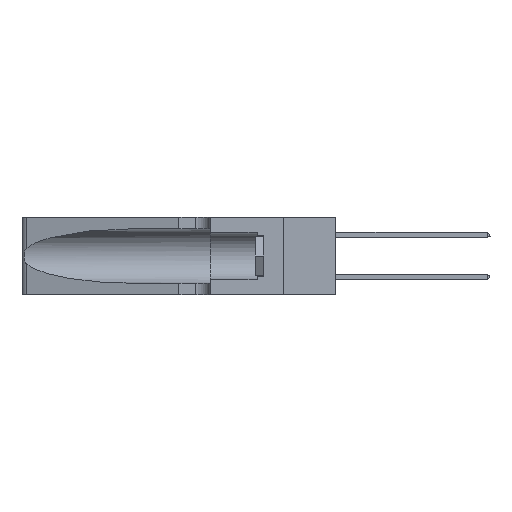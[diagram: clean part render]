
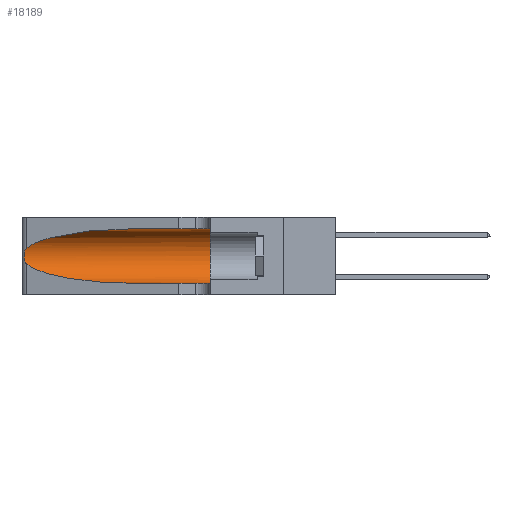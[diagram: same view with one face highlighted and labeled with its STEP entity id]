
A CAD part, left-side view. The second image highlights one B-rep face of the part: STEP entity #18189.
In plain terms, the highlighted cylindrical face has radius 3.308 mm (diameter 6.617 mm), a partial arc.
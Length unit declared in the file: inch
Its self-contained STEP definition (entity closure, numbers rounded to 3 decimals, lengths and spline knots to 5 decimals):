
#1156 = VECTOR ( 'NONE', #6604, 39.37008 ) ;
#1257 = CARTESIAN_POINT ( 'NONE',  ( 0.25789, 1.23486, 0.15765 ) ) ;
#1848 = CARTESIAN_POINT ( 'NONE',  ( 0.1305, 0.72297, 0.31525 ) ) ;
#2786 = EDGE_CURVE ( 'NONE', #25239, #17567, #21414, .T. ) ;
#2824 = CARTESIAN_POINT ( 'NONE',  ( 0.2373, 1.15595, 0.08982 ) ) ;
#3419 = CARTESIAN_POINT ( 'NONE',  ( 0.25555, 1.22993, 0.14849 ) ) ;
#3692 = CARTESIAN_POINT ( 'NONE',  ( 0.25854, 1.2359, 0.20912 ) ) ;
#4464 = B_SPLINE_CURVE_WITH_KNOTS ( 'NONE', 3,
 ( #20615, #18789, #14091, #18620, #3692, #5866, #8027, #5594, #10158, #25153, #1257, #7849, #3419, #18433 ),
 .UNSPECIFIED., .F., .F.,
 ( 4, 2, 2, 2, 2, 2, 4 ),
 ( 0., 0.00027, 0.00053, 0.00107, 0.0016, 0.00187, 0.00214 ),
 .UNSPECIFIED. ) ;
#4589 = ORIENTED_EDGE ( 'NONE', *, *, #23152, .T. ) ;
#4633 = VERTEX_POINT ( 'NONE', #17608 ) ;
#4641 = EDGE_CURVE ( 'NONE', #10341, #25239, #5870, .T. ) ;
#4754 = DIRECTION ( 'NONE',  ( 0., -1., 0. ) ) ;
#5594 = CARTESIAN_POINT ( 'NONE',  ( 0.26075, 1.23896, 0.178 ) ) ;
#5866 = CARTESIAN_POINT ( 'NONE',  ( 0.26018, 1.23835, 0.19895 ) ) ;
#5870 = LINE ( 'NONE', #19462, #1156 ) ;
#6142 = CARTESIAN_POINT ( 'NONE',  ( 0.2373, 1.15595, 0.28018 ) ) ;
#6604 = DIRECTION ( 'NONE',  ( 0., -1., 0. ) ) ;
#6938 = DIRECTION ( 'NONE',  ( 0., -1., 0. ) ) ;
#7849 = CARTESIAN_POINT ( 'NONE',  ( 0.25639, 1.23186, 0.15144 ) ) ;
#8027 = CARTESIAN_POINT ( 'NONE',  ( 0.26075, 1.23896, 0.19203 ) ) ;
#8057 = CYLINDRICAL_SURFACE ( 'NONE', #11708, 0.13025 ) ;
#8384 = CARTESIAN_POINT ( 'NONE',  ( 0.25487, 1.22718, 0.22369 ) ) ;
#8894 = CARTESIAN_POINT ( 'NONE',  ( 0.1305, 1.61858, 0.185 ) ) ;
#8981 = DIRECTION ( 'NONE',  ( 0., 0., -1. ) ) ;
#9830 = CARTESIAN_POINT ( 'NONE',  ( 0.1305, 0.72297, 0.05475 ) ) ;
#10158 = CARTESIAN_POINT ( 'NONE',  ( 0.26017, 1.23833, 0.17102 ) ) ;
#10341 = VERTEX_POINT ( 'NONE', #1848 ) ;
#10532 = CARTESIAN_POINT ( 'NONE',  ( 0.1305, 0.72297, 0.31525 ) ) ;
#10904 = CARTESIAN_POINT ( 'NONE',  ( 0.25487, 1.22718, 0.22369 ) ) ;
#11274 = CARTESIAN_POINT ( 'NONE',  ( 0.25487, 1.22718, 0.14631 ) ) ;
#11298 = LINE ( 'NONE', #26339, #27071 ) ;
#11708 = AXIS2_PLACEMENT_3D ( 'NONE', #8894, #4754, #8981 ) ;
#12386 = AXIS2_PLACEMENT_3D ( 'NONE', #13321, #15680, #17861 ) ;
#13321 = CARTESIAN_POINT ( 'NONE',  ( 0.1305, 0.35, 0.185 ) ) ;
#14091 = CARTESIAN_POINT ( 'NONE',  ( 0.25639, 1.23184, 0.21858 ) ) ;
#14952 = CARTESIAN_POINT ( 'NONE',  ( 0.18966, 0.96281, 0.31525 ) ) ;
#15680 = DIRECTION ( 'NONE',  ( 0., 1., 0. ) ) ;
#16742 = EDGE_CURVE ( 'NONE', #4633, #17568, #27338, .T. ) ;
#17567 = VERTEX_POINT ( 'NONE', #24806 ) ;
#17568 = VERTEX_POINT ( 'NONE', #9830 ) ;
#17608 = CARTESIAN_POINT ( 'NONE',  ( 0.25487, 1.22718, 0.14631 ) ) ;
#17740 = ORIENTED_EDGE ( 'NONE', *, *, #26676, .T. ) ;
#17861 = DIRECTION ( 'NONE',  ( 0., 0., 1. ) ) ;
#18189 = ADVANCED_FACE ( 'NONE', ( #27170 ), #8057, .F. ) ;
#18433 = CARTESIAN_POINT ( 'NONE',  ( 0.25487, 1.22718, 0.14631 ) ) ;
#18620 = CARTESIAN_POINT ( 'NONE',  ( 0.25787, 1.23484, 0.2124 ) ) ;
#18789 = CARTESIAN_POINT ( 'NONE',  ( 0.25555, 1.22994, 0.2215 ) ) ;
#19434 =( BOUNDED_CURVE ( )  B_SPLINE_CURVE ( 3, ( #10532, #14952, #6142, #8384 ),
 .UNSPECIFIED., .F., .F. ) 
 B_SPLINE_CURVE_WITH_KNOTS ( ( 4, 4 ),
 ( 1.5708, 2.84003 ),
 .UNSPECIFIED. ) 
 CURVE ( )  GEOMETRIC_REPRESENTATION_ITEM ( )  RATIONAL_B_SPLINE_CURVE ( ( 1., 0.87, 0.87, 1. ) ) 
 REPRESENTATION_ITEM ( '' )  );
#19462 = CARTESIAN_POINT ( 'NONE',  ( 0.1305, 1.61858, 0.31525 ) ) ;
#20203 = EDGE_CURVE ( 'NONE', #17568, #17567, #11298, .T. ) ;
#20615 = CARTESIAN_POINT ( 'NONE',  ( 0.25487, 1.22718, 0.22369 ) ) ;
#21414 = CIRCLE ( 'NONE', #12386, 0.13025 ) ;
#21694 = CARTESIAN_POINT ( 'NONE',  ( 0.1305, 0.72297, 0.05475 ) ) ;
#22154 = ORIENTED_EDGE ( 'NONE', *, *, #2786, .F. ) ;
#22510 = CARTESIAN_POINT ( 'NONE',  ( 0.1305, 0.35, 0.31525 ) ) ;
#22972 = ORIENTED_EDGE ( 'NONE', *, *, #20203, .T. ) ;
#23152 = EDGE_CURVE ( 'NONE', #23429, #4633, #4464, .T. ) ;
#23429 = VERTEX_POINT ( 'NONE', #10904 ) ;
#23927 = CARTESIAN_POINT ( 'NONE',  ( 0.18966, 0.96281, 0.05475 ) ) ;
#24346 = EDGE_LOOP ( 'NONE', ( #17740, #4589, #25095, #22972, #22154, #26927 ) ) ;
#24806 = CARTESIAN_POINT ( 'NONE',  ( 0.1305, 0.35, 0.05475 ) ) ;
#25095 = ORIENTED_EDGE ( 'NONE', *, *, #16742, .T. ) ;
#25153 = CARTESIAN_POINT ( 'NONE',  ( 0.25856, 1.23593, 0.16098 ) ) ;
#25239 = VERTEX_POINT ( 'NONE', #22510 ) ;
#26339 = CARTESIAN_POINT ( 'NONE',  ( 0.1305, 1.61858, 0.05475 ) ) ;
#26676 = EDGE_CURVE ( 'NONE', #10341, #23429, #19434, .T. ) ;
#26927 = ORIENTED_EDGE ( 'NONE', *, *, #4641, .F. ) ;
#27071 = VECTOR ( 'NONE', #6938, 39.37008 ) ;
#27170 = FACE_OUTER_BOUND ( 'NONE', #24346, .T. ) ;
#27338 =( BOUNDED_CURVE ( )  B_SPLINE_CURVE ( 3, ( #11274, #2824, #23927, #21694 ),
 .UNSPECIFIED., .F., .F. ) 
 B_SPLINE_CURVE_WITH_KNOTS ( ( 4, 4 ),
 ( 3.44316, 4.71239 ),
 .UNSPECIFIED. ) 
 CURVE ( )  GEOMETRIC_REPRESENTATION_ITEM ( )  RATIONAL_B_SPLINE_CURVE ( ( 1., 0.87, 0.87, 1. ) ) 
 REPRESENTATION_ITEM ( '' )  );
